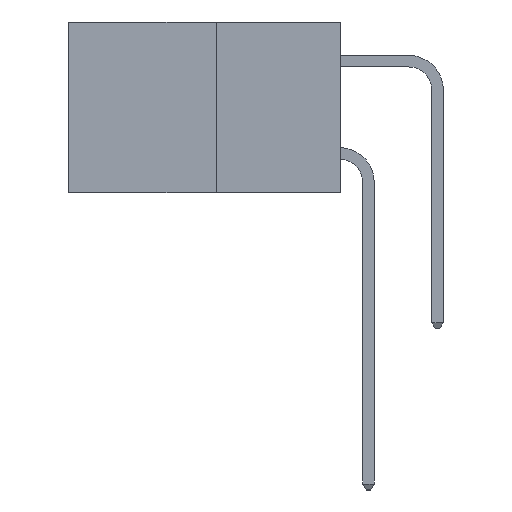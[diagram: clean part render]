
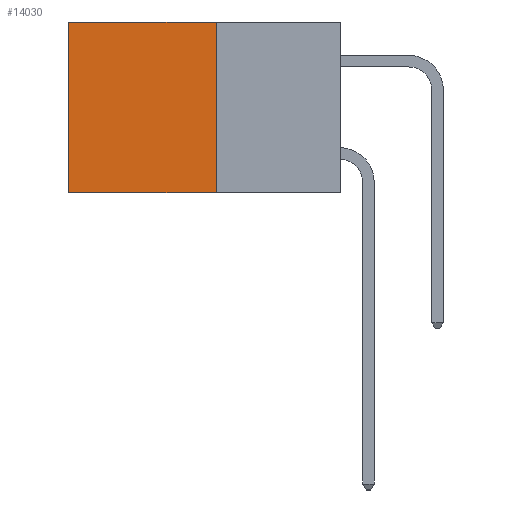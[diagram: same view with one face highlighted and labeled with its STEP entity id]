
A CAD part, left-side view. The second image highlights one B-rep face of the part: STEP entity #14030.
In plain terms, the highlighted planar face has unit normal (-1, 0, 0).
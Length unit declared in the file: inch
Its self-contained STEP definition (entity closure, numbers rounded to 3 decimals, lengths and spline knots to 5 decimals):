
#2095 = VECTOR ( 'NONE', #9002, 39.37008 ) ;
#2183 = ORIENTED_EDGE ( 'NONE', *, *, #11464, .F. ) ;
#2440 = VECTOR ( 'NONE', #12859, 39.37008 ) ;
#2822 = CARTESIAN_POINT ( 'NONE',  ( 0.277, 0.27, 0. ) ) ;
#2982 = EDGE_CURVE ( 'NONE', #5561, #6643, #10306, .T. ) ;
#3111 = CARTESIAN_POINT ( 'NONE',  ( 0.277, 0.27, -0.37 ) ) ;
#3415 = CARTESIAN_POINT ( 'NONE',  ( 0.277, 0.59, 0. ) ) ;
#3582 = PLANE ( 'NONE',  #6451 ) ;
#3658 = DIRECTION ( 'NONE',  ( 0., 1., 0. ) ) ;
#4420 = CARTESIAN_POINT ( 'NONE',  ( 0.277, 0.59, -0.37 ) ) ;
#4492 = EDGE_CURVE ( 'NONE', #6643, #13883, #4977, .T. ) ;
#4635 = EDGE_CURVE ( 'NONE', #5561, #6944, #5348, .T. ) ;
#4977 = LINE ( 'NONE', #14655, #7026 ) ;
#5348 = LINE ( 'NONE', #7984, #2095 ) ;
#5561 = VERTEX_POINT ( 'NONE', #9244 ) ;
#6451 = AXIS2_PLACEMENT_3D ( 'NONE', #10433, #13863, #7024 ) ;
#6643 = VERTEX_POINT ( 'NONE', #3415 ) ;
#6944 = VERTEX_POINT ( 'NONE', #3111 ) ;
#7024 = DIRECTION ( 'NONE',  ( 0., 0., -1. ) ) ;
#7026 = VECTOR ( 'NONE', #8896, 39.37008 ) ;
#7140 = ORIENTED_EDGE ( 'NONE', *, *, #4635, .F. ) ;
#7984 = CARTESIAN_POINT ( 'NONE',  ( 0.277, 0.27, -0.37 ) ) ;
#8896 = DIRECTION ( 'NONE',  ( 0., 0., -1. ) ) ;
#9002 = DIRECTION ( 'NONE',  ( 0., 0., -1. ) ) ;
#9244 = CARTESIAN_POINT ( 'NONE',  ( 0.277, 0.27, 0. ) ) ;
#9706 = ORIENTED_EDGE ( 'NONE', *, *, #4492, .T. ) ;
#10306 = LINE ( 'NONE', #2822, #12978 ) ;
#10433 = CARTESIAN_POINT ( 'NONE',  ( 0.277, 0.27, -0.37 ) ) ;
#10498 = EDGE_LOOP ( 'NONE', ( #9706, #2183, #7140, #14822 ) ) ;
#11464 = EDGE_CURVE ( 'NONE', #6944, #13883, #11513, .T. ) ;
#11513 = LINE ( 'NONE', #11709, #2440 ) ;
#11709 = CARTESIAN_POINT ( 'NONE',  ( 0.277, 0.27, -0.37 ) ) ;
#12859 = DIRECTION ( 'NONE',  ( 0., 1., 0. ) ) ;
#12978 = VECTOR ( 'NONE', #3658, 39.37008 ) ;
#13307 = FACE_OUTER_BOUND ( 'NONE', #10498, .T. ) ;
#13863 = DIRECTION ( 'NONE',  ( 1., 0., 0. ) ) ;
#13883 = VERTEX_POINT ( 'NONE', #4420 ) ;
#14030 = ADVANCED_FACE ( 'NONE', ( #13307 ), #3582, .F. ) ;
#14655 = CARTESIAN_POINT ( 'NONE',  ( 0.277, 0.59, -0.37 ) ) ;
#14822 = ORIENTED_EDGE ( 'NONE', *, *, #2982, .T. ) ;
